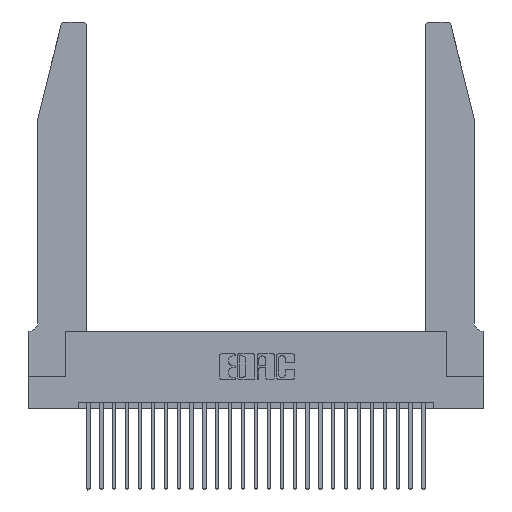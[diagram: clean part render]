
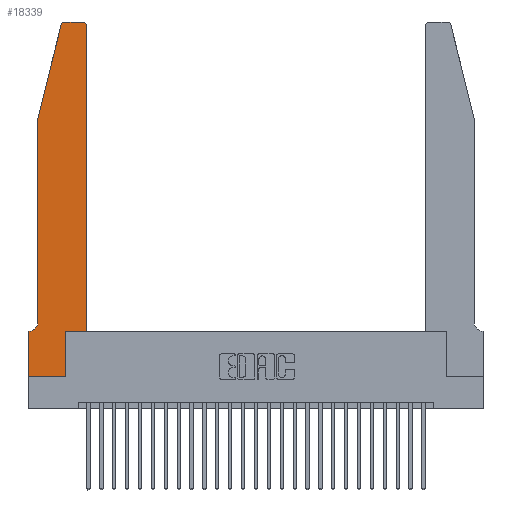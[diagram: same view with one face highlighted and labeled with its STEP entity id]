
A CAD part, top view. The second image highlights one B-rep face of the part: STEP entity #18339.
In plain terms, the highlighted planar face has unit normal (0, 0, 1).
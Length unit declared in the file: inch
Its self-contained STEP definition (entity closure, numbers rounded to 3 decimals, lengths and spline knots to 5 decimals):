
#444 = DIRECTION ( 'NONE',  ( 0., 0., -1. ) ) ;
#618 = VERTEX_POINT ( 'NONE', #20405 ) ;
#1477 = DIRECTION ( 'NONE',  ( -1., 0., 0. ) ) ;
#1510 = VECTOR ( 'NONE', #2868, 39.37008 ) ;
#2236 = EDGE_CURVE ( 'NONE', #3885, #618, #27696, .T. ) ;
#2295 = VERTEX_POINT ( 'NONE', #24138 ) ;
#2771 = CARTESIAN_POINT ( 'NONE',  ( 0.0755, 2., 0.37 ) ) ;
#2868 = DIRECTION ( 'NONE',  ( -0.239, -0.971, 0. ) ) ;
#3253 = VECTOR ( 'NONE', #19387, 39.37008 ) ;
#3885 = VERTEX_POINT ( 'NONE', #4042 ) ;
#4042 = CARTESIAN_POINT ( 'NONE',  ( 0.0755, 0.42, 0.37 ) ) ;
#4545 = DIRECTION ( 'NONE',  ( 0., 0., 1. ) ) ;
#4603 = CARTESIAN_POINT ( 'NONE',  ( 0.0055, 0.42, 0.37 ) ) ;
#4696 = CARTESIAN_POINT ( 'NONE',  ( 0., 0., 0.37 ) ) ;
#5506 = LINE ( 'NONE', #23902, #24769 ) ;
#5980 = LINE ( 'NONE', #15155, #3253 ) ;
#6139 = EDGE_CURVE ( 'NONE', #23951, #2295, #8941, .T. ) ;
#6228 = VECTOR ( 'NONE', #27609, 39.37008 ) ;
#6326 = CIRCLE ( 'NONE', #18176, 0.03 ) ;
#6547 = ORIENTED_EDGE ( 'NONE', *, *, #25296, .T. ) ;
#6558 = CARTESIAN_POINT ( 'NONE',  ( 0.0755, 2., 0.37 ) ) ;
#6675 = EDGE_CURVE ( 'NONE', #7029, #14087, #11984, .T. ) ;
#6922 = DIRECTION ( 'NONE',  ( 0., -1., 0. ) ) ;
#6926 = EDGE_CURVE ( 'NONE', #618, #23951, #16970, .T. ) ;
#7029 = VERTEX_POINT ( 'NONE', #18512 ) ;
#7712 = ORIENTED_EDGE ( 'NONE', *, *, #12967, .T. ) ;
#8173 = LINE ( 'NONE', #19030, #13905 ) ;
#8295 = CARTESIAN_POINT ( 'NONE',  ( 0., 0.35, 0.37 ) ) ;
#8454 = CARTESIAN_POINT ( 'NONE',  ( 0.4205, 2.75, 0.37 ) ) ;
#8894 = EDGE_CURVE ( 'NONE', #15976, #24021, #27521, .T. ) ;
#8941 = LINE ( 'NONE', #4696, #13008 ) ;
#9016 = ORIENTED_EDGE ( 'NONE', *, *, #6926, .T. ) ;
#9353 = LINE ( 'NONE', #19294, #22138 ) ;
#9566 = CARTESIAN_POINT ( 'NONE',  ( 0.2865, 0.35, 0.37 ) ) ;
#10564 = AXIS2_PLACEMENT_3D ( 'NONE', #27972, #23606, #25709 ) ;
#11984 = LINE ( 'NONE', #23139, #6228 ) ;
#12452 = CARTESIAN_POINT ( 'NONE',  ( 0.0755, 0.35, 0.37 ) ) ;
#12967 = EDGE_CURVE ( 'NONE', #2295, #24903, #5980, .T. ) ;
#13008 = VECTOR ( 'NONE', #26633, 39.37008 ) ;
#13318 = DIRECTION ( 'NONE',  ( -1., 0., 0. ) ) ;
#13494 = FACE_OUTER_BOUND ( 'NONE', #18645, .T. ) ;
#13620 = ORIENTED_EDGE ( 'NONE', *, *, #23376, .T. ) ;
#13905 = VECTOR ( 'NONE', #18841, 39.37008 ) ;
#14087 = VERTEX_POINT ( 'NONE', #14359 ) ;
#14208 = EDGE_CURVE ( 'NONE', #21686, #20437, #6326, .T. ) ;
#14359 = CARTESIAN_POINT ( 'NONE',  ( 0.4505, 0.35, 0.37 ) ) ;
#14701 = ORIENTED_EDGE ( 'NONE', *, *, #2236, .T. ) ;
#14947 = AXIS2_PLACEMENT_3D ( 'NONE', #26009, #4545, #15324 ) ;
#15155 = CARTESIAN_POINT ( 'NONE',  ( 0., 0., 0.37 ) ) ;
#15324 = DIRECTION ( 'NONE',  ( 1., 0., 0. ) ) ;
#15849 = DIRECTION ( 'NONE',  ( 0., 1., 0. ) ) ;
#15976 = VERTEX_POINT ( 'NONE', #19712 ) ;
#16060 = VECTOR ( 'NONE', #15849, 39.37008 ) ;
#16364 = VERTEX_POINT ( 'NONE', #27752 ) ;
#16655 = ORIENTED_EDGE ( 'NONE', *, *, #19830, .T. ) ;
#16970 = LINE ( 'NONE', #12452, #25462 ) ;
#17047 = ORIENTED_EDGE ( 'NONE', *, *, #6139, .T. ) ;
#17382 = DIRECTION ( 'NONE',  ( -1., 0., 0. ) ) ;
#17801 = ORIENTED_EDGE ( 'NONE', *, *, #22266, .T. ) ;
#18176 = AXIS2_PLACEMENT_3D ( 'NONE', #21587, #21304, #19138 ) ;
#18339 = ADVANCED_FACE ( 'NONE', ( #13494 ), #25896, .T. ) ;
#18512 = CARTESIAN_POINT ( 'NONE',  ( 0.2865, 0.35, 0.37 ) ) ;
#18645 = EDGE_LOOP ( 'NONE', ( #16655, #17801, #22681, #23056, #14701, #9016, #17047, #7712, #6547, #20943, #13620, #27810 ) ) ;
#18841 = DIRECTION ( 'NONE',  ( 0., 1., 0. ) ) ;
#19030 = CARTESIAN_POINT ( 'NONE',  ( 0.4505, 0.35, 0.37 ) ) ;
#19138 = DIRECTION ( 'NONE',  ( 1., 0., 0. ) ) ;
#19294 = CARTESIAN_POINT ( 'NONE',  ( 0.2605, 2.75, 0.37 ) ) ;
#19387 = DIRECTION ( 'NONE',  ( 1., 0., 0. ) ) ;
#19712 = CARTESIAN_POINT ( 'NONE',  ( 0.25487, 2.72718, 0.37 ) ) ;
#19830 = EDGE_CURVE ( 'NONE', #20437, #16364, #9353, .T. ) ;
#20405 = CARTESIAN_POINT ( 'NONE',  ( 0.0055, 0.35, 0.37 ) ) ;
#20437 = VERTEX_POINT ( 'NONE', #8454 ) ;
#20542 = AXIS2_PLACEMENT_3D ( 'NONE', #4603, #444, #13318 ) ;
#20611 = CARTESIAN_POINT ( 'NONE',  ( 0.4505, 2.72, 0.37 ) ) ;
#20943 = ORIENTED_EDGE ( 'NONE', *, *, #6675, .T. ) ;
#21304 = DIRECTION ( 'NONE',  ( 0., 0., 1. ) ) ;
#21587 = CARTESIAN_POINT ( 'NONE',  ( 0.4205, 2.72, 0.37 ) ) ;
#21686 = VERTEX_POINT ( 'NONE', #20611 ) ;
#22138 = VECTOR ( 'NONE', #17382, 39.37008 ) ;
#22182 = EDGE_CURVE ( 'NONE', #24021, #3885, #5506, .T. ) ;
#22266 = EDGE_CURVE ( 'NONE', #16364, #15976, #23731, .T. ) ;
#22681 = ORIENTED_EDGE ( 'NONE', *, *, #8894, .T. ) ;
#23056 = ORIENTED_EDGE ( 'NONE', *, *, #22182, .T. ) ;
#23139 = CARTESIAN_POINT ( 'NONE',  ( 0.4505, 0.35, 0.37 ) ) ;
#23376 = EDGE_CURVE ( 'NONE', #14087, #21686, #8173, .T. ) ;
#23606 = DIRECTION ( 'NONE',  ( 0., 0., 1. ) ) ;
#23731 = CIRCLE ( 'NONE', #14947, 0.03 ) ;
#23902 = CARTESIAN_POINT ( 'NONE',  ( 0.0755, 2., 0.37 ) ) ;
#23951 = VERTEX_POINT ( 'NONE', #8295 ) ;
#24021 = VERTEX_POINT ( 'NONE', #6558 ) ;
#24138 = CARTESIAN_POINT ( 'NONE',  ( 0., 0., 0.37 ) ) ;
#24769 = VECTOR ( 'NONE', #6922, 39.37008 ) ;
#24903 = VERTEX_POINT ( 'NONE', #26544 ) ;
#25296 = EDGE_CURVE ( 'NONE', #24903, #7029, #25914, .T. ) ;
#25462 = VECTOR ( 'NONE', #1477, 39.37008 ) ;
#25709 = DIRECTION ( 'NONE',  ( 1., 0., 0. ) ) ;
#25896 = PLANE ( 'NONE',  #10564 ) ;
#25914 = LINE ( 'NONE', #9566, #16060 ) ;
#26009 = CARTESIAN_POINT ( 'NONE',  ( 0.284, 2.72, 0.37 ) ) ;
#26544 = CARTESIAN_POINT ( 'NONE',  ( 0.2865, 0., 0.37 ) ) ;
#26633 = DIRECTION ( 'NONE',  ( 0., -1., 0. ) ) ;
#27521 = LINE ( 'NONE', #2771, #1510 ) ;
#27609 = DIRECTION ( 'NONE',  ( 1., 0., 0. ) ) ;
#27696 = CIRCLE ( 'NONE', #20542, 0.07 ) ;
#27752 = CARTESIAN_POINT ( 'NONE',  ( 0.284, 2.75, 0.37 ) ) ;
#27810 = ORIENTED_EDGE ( 'NONE', *, *, #14208, .T. ) ;
#27972 = CARTESIAN_POINT ( 'NONE',  ( 0., 0.35, 0.37 ) ) ;
